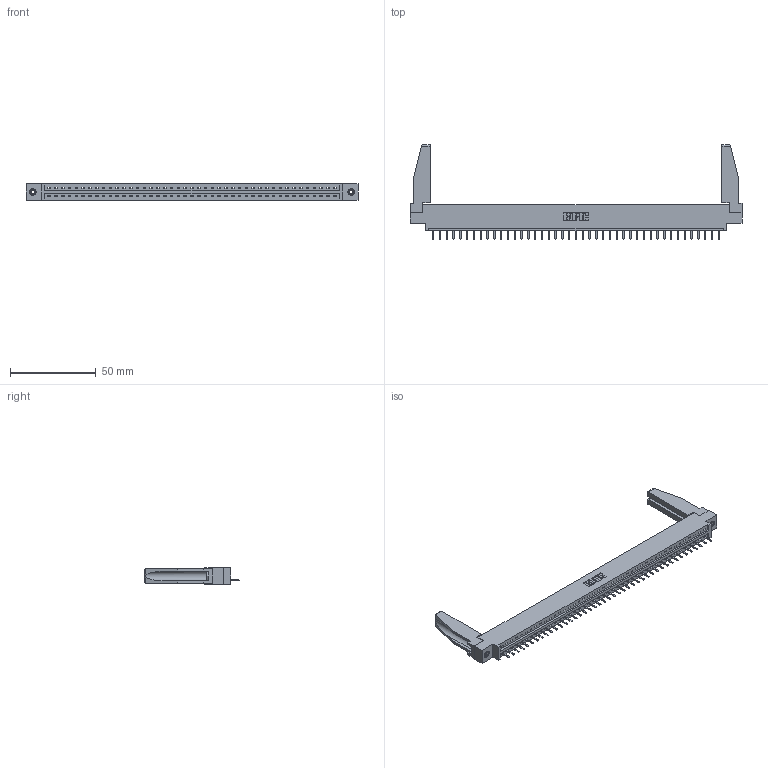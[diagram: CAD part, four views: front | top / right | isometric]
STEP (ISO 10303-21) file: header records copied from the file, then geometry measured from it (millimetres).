
FILE_DESCRIPTION (( 'STEP AP203' ), '1' );
FILE_NAME ('387-043-520-678.STEP', '2019-10-04T21:44:23', ( '' ), ( '' ), 'SwSTEP 2.0', 'SolidWorks 2016', '' );
FILE_SCHEMA (( 'CONFIG_CONTROL_DESIGN' ));
Length unit declared in the file: inch
Products named in the file (5): 387-043-520-678; 307-220-078; 345-250-001_345-250-001-102; 337 Part_0.170 Offset - 0.156 Dia-TI; 345-292-001_345-293-120
Assembly tree (48 placements, depth 2):
  387-043-520-678
    337 Part_0.170 Offset - 0.156 Dia-TI
    345-292-001_345-293-120  x43
    345-250-001_345-250-001-102  x2
    307-220-078  x2
Bounding box: 193.4 x 54.82 x 9.4 mm (x, y, z)
Volume: 23864.9 mm3; surface area: 24027.9 mm2
Topology: 48 solids, 48 shells, 3086 faces, 9081 edges, 5930 vertices
Faces by surface type: plane 2222, cylinder 848, cone 12, torus 4
Entity records: 34520 total; most frequent: CARTESIAN_POINT 6017, ORIENTED_EDGE 5940, DIRECTION 5060, EDGE_CURVE 2970, LINE 2800, VECTOR 2800, VERTEX_POINT 1972, AXIS2_PLACEMENT_3D 1130
